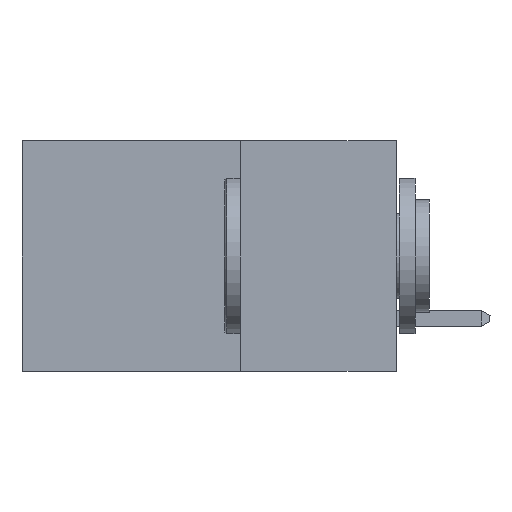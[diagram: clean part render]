
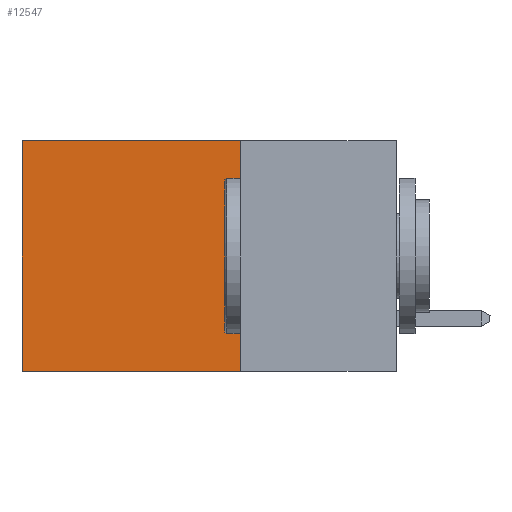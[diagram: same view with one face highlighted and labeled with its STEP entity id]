
A CAD part, left-side view. The second image highlights one B-rep face of the part: STEP entity #12547.
In plain terms, the highlighted planar face has unit normal (-1, 0, 0).
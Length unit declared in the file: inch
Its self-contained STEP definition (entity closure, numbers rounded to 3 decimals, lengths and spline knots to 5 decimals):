
#1003 = PLANE ( 'NONE',  #9458 ) ;
#1172 = VECTOR ( 'NONE', #3858, 39.37008 ) ;
#1538 = LINE ( 'NONE', #3623, #1172 ) ;
#1844 = LINE ( 'NONE', #10193, #2182 ) ;
#2005 = VECTOR ( 'NONE', #6505, 39.37008 ) ;
#2182 = VECTOR ( 'NONE', #10334, 39.37008 ) ;
#2302 = CARTESIAN_POINT ( 'NONE',  ( 0.2615, 0.25, 0. ) ) ;
#2834 = ORIENTED_EDGE ( 'NONE', *, *, #3454, .T. ) ;
#2872 = CARTESIAN_POINT ( 'NONE',  ( 0.2615, 0.6, -0.37 ) ) ;
#3011 = ORIENTED_EDGE ( 'NONE', *, *, #4731, .F. ) ;
#3093 = ORIENTED_EDGE ( 'NONE', *, *, #3440, .F. ) ;
#3189 = CARTESIAN_POINT ( 'NONE',  ( 0.2615, 0.6, -0.37 ) ) ;
#3217 = DIRECTION ( 'NONE',  ( 0., 0., -1. ) ) ;
#3281 = VERTEX_POINT ( 'NONE', #6218 ) ;
#3320 = ORIENTED_EDGE ( 'NONE', *, *, #10833, .T. ) ;
#3440 = EDGE_CURVE ( 'NONE', #4978, #3281, #1538, .T. ) ;
#3454 = EDGE_CURVE ( 'NONE', #10765, #3477, #6247, .T. ) ;
#3477 = VERTEX_POINT ( 'NONE', #2872 ) ;
#3478 = CARTESIAN_POINT ( 'NONE',  ( 0.2615, 0.6, 0. ) ) ;
#3623 = CARTESIAN_POINT ( 'NONE',  ( 0.2615, 0.25, -0.37 ) ) ;
#3858 = DIRECTION ( 'NONE',  ( 0., 0., -1. ) ) ;
#4354 = LINE ( 'NONE', #10362, #2005 ) ;
#4731 = EDGE_CURVE ( 'NONE', #3281, #3477, #1844, .T. ) ;
#4978 = VERTEX_POINT ( 'NONE', #2302 ) ;
#5088 = DIRECTION ( 'NONE',  ( 0., 0., -1. ) ) ;
#6218 = CARTESIAN_POINT ( 'NONE',  ( 0.2615, 0.25, -0.37 ) ) ;
#6247 = LINE ( 'NONE', #3189, #6524 ) ;
#6505 = DIRECTION ( 'NONE',  ( 0., 1., 0. ) ) ;
#6524 = VECTOR ( 'NONE', #3217, 39.37008 ) ;
#8012 = CARTESIAN_POINT ( 'NONE',  ( 0.2615, 0.25, -0.37 ) ) ;
#9458 = AXIS2_PLACEMENT_3D ( 'NONE', #8012, #10888, #5088 ) ;
#9946 = EDGE_LOOP ( 'NONE', ( #2834, #3011, #3093, #3320 ) ) ;
#10193 = CARTESIAN_POINT ( 'NONE',  ( 0.2615, 0.25, -0.37 ) ) ;
#10241 = FACE_OUTER_BOUND ( 'NONE', #9946, .T. ) ;
#10334 = DIRECTION ( 'NONE',  ( 0., 1., 0. ) ) ;
#10362 = CARTESIAN_POINT ( 'NONE',  ( 0.2615, 0.25, 0. ) ) ;
#10765 = VERTEX_POINT ( 'NONE', #3478 ) ;
#10833 = EDGE_CURVE ( 'NONE', #4978, #10765, #4354, .T. ) ;
#10888 = DIRECTION ( 'NONE',  ( 1., 0., 0. ) ) ;
#12547 = ADVANCED_FACE ( 'NONE', ( #10241 ), #1003, .F. ) ;
